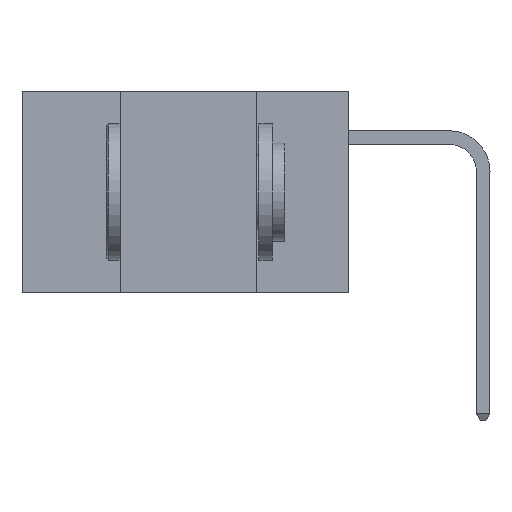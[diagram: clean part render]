
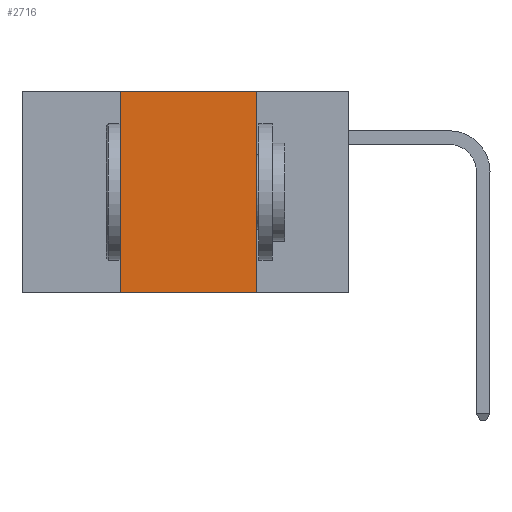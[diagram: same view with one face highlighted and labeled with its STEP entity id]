
A CAD part, left-side view. The second image highlights one B-rep face of the part: STEP entity #2716.
In plain terms, the highlighted planar face has unit normal (-1, 0, 0).
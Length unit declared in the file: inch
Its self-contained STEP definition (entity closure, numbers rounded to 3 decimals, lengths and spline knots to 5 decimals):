
#550 = LINE ( 'NONE', #14141, #15633 ) ;
#840 = CARTESIAN_POINT ( 'NONE',  ( 0., 0.17, 0. ) ) ;
#907 = ORIENTED_EDGE ( 'NONE', *, *, #8487, .F. ) ;
#1345 = CARTESIAN_POINT ( 'NONE',  ( 0., 0.6, 0. ) ) ;
#1838 = ORIENTED_EDGE ( 'NONE', *, *, #15477, .F. ) ;
#2555 = CARTESIAN_POINT ( 'NONE',  ( 0., 0.17, -0.37 ) ) ;
#2640 = ORIENTED_EDGE ( 'NONE', *, *, #8449, .T. ) ;
#2716 = ADVANCED_FACE ( 'NONE', ( #7753 ), #10006, .F. ) ;
#3440 = CARTESIAN_POINT ( 'NONE',  ( 0., 0.6, -0.37 ) ) ;
#3469 = DIRECTION ( 'NONE',  ( 0., -1., 0. ) ) ;
#4524 = LINE ( 'NONE', #3440, #5280 ) ;
#4740 = LINE ( 'NONE', #840, #10569 ) ;
#5280 = VECTOR ( 'NONE', #13082, 39.37008 ) ;
#5657 = VECTOR ( 'NONE', #8109, 39.37008 ) ;
#5810 = CARTESIAN_POINT ( 'NONE',  ( 0., 0.42, 0. ) ) ;
#5972 = ORIENTED_EDGE ( 'NONE', *, *, #7850, .F. ) ;
#6303 = AXIS2_PLACEMENT_3D ( 'NONE', #1345, #8763, #11030 ) ;
#7753 = FACE_OUTER_BOUND ( 'NONE', #9570, .T. ) ;
#7850 = EDGE_CURVE ( 'NONE', #9626, #10762, #4740, .T. ) ;
#8109 = DIRECTION ( 'NONE',  ( 0., 0., 1. ) ) ;
#8424 = VERTEX_POINT ( 'NONE', #5810 ) ;
#8449 = EDGE_CURVE ( 'NONE', #10153, #10762, #4524, .T. ) ;
#8487 = EDGE_CURVE ( 'NONE', #10153, #8424, #10573, .T. ) ;
#8763 = DIRECTION ( 'NONE',  ( 1., 0., 0. ) ) ;
#9193 = DIRECTION ( 'NONE',  ( 0., 0., -1. ) ) ;
#9570 = EDGE_LOOP ( 'NONE', ( #5972, #1838, #907, #2640 ) ) ;
#9626 = VERTEX_POINT ( 'NONE', #10384 ) ;
#10006 = PLANE ( 'NONE',  #6303 ) ;
#10153 = VERTEX_POINT ( 'NONE', #12822 ) ;
#10384 = CARTESIAN_POINT ( 'NONE',  ( 0., 0.17, 0. ) ) ;
#10569 = VECTOR ( 'NONE', #9193, 39.37008 ) ;
#10573 = LINE ( 'NONE', #11677, #5657 ) ;
#10762 = VERTEX_POINT ( 'NONE', #2555 ) ;
#11030 = DIRECTION ( 'NONE',  ( 0., 0., -1. ) ) ;
#11677 = CARTESIAN_POINT ( 'NONE',  ( 0., 0.42, 0. ) ) ;
#12822 = CARTESIAN_POINT ( 'NONE',  ( 0., 0.42, -0.37 ) ) ;
#13082 = DIRECTION ( 'NONE',  ( 0., -1., 0. ) ) ;
#14141 = CARTESIAN_POINT ( 'NONE',  ( 0., 0.6, 0. ) ) ;
#15477 = EDGE_CURVE ( 'NONE', #8424, #9626, #550, .T. ) ;
#15633 = VECTOR ( 'NONE', #3469, 39.37008 ) ;
